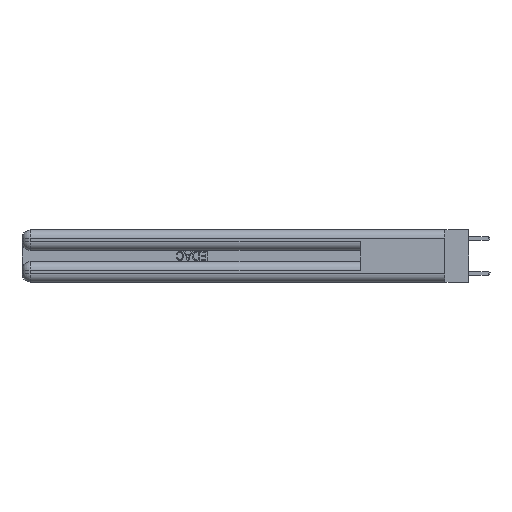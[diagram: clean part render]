
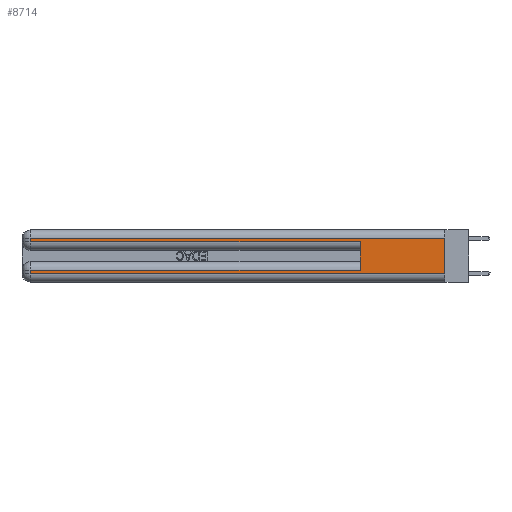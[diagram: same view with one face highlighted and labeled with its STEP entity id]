
A CAD part, left-side view. The second image highlights one B-rep face of the part: STEP entity #8714.
In plain terms, the highlighted planar face has unit normal (-1, 0, 0).
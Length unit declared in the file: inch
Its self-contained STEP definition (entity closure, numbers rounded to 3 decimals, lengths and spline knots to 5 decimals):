
#785 = CARTESIAN_POINT ( 'NONE',  ( 0., 0.6, 0.085 ) ) ;
#1132 = LINE ( 'NONE', #3684, #12643 ) ;
#1412 = CARTESIAN_POINT ( 'NONE',  ( 0., 2.94, 0.31 ) ) ;
#2000 = CARTESIAN_POINT ( 'NONE',  ( 0., 0., 0.31 ) ) ;
#2196 = DIRECTION ( 'NONE',  ( 0., -1., 0. ) ) ;
#3432 = CARTESIAN_POINT ( 'NONE',  ( 0., 0., 0.31 ) ) ;
#3684 = CARTESIAN_POINT ( 'NONE',  ( 0., 0., 0.06 ) ) ;
#5345 = EDGE_CURVE ( 'NONE', #19648, #17023, #16332, .T. ) ;
#5467 = DIRECTION ( 'NONE',  ( 1., 0., 0. ) ) ;
#5816 = DIRECTION ( 'NONE',  ( 0., 0., -1. ) ) ;
#6574 = AXIS2_PLACEMENT_3D ( 'NONE', #23707, #5467, #21513 ) ;
#6749 = CARTESIAN_POINT ( 'NONE',  ( 0., 0., 0.285 ) ) ;
#7258 = VERTEX_POINT ( 'NONE', #28825 ) ;
#8148 = VERTEX_POINT ( 'NONE', #28732 ) ;
#8714 = ADVANCED_FACE ( 'NONE', ( #24855 ), #19241, .F. ) ;
#8720 = CARTESIAN_POINT ( 'NONE',  ( 0., 2.94, 0.37 ) ) ;
#9172 = VECTOR ( 'NONE', #20385, 39.37008 ) ;
#9452 = VERTEX_POINT ( 'NONE', #3432 ) ;
#10529 = VECTOR ( 'NONE', #26042, 39.37008 ) ;
#10895 = CARTESIAN_POINT ( 'NONE',  ( 0., 0.6, 0.145 ) ) ;
#11753 = EDGE_CURVE ( 'NONE', #17023, #7258, #26459, .T. ) ;
#12235 = EDGE_CURVE ( 'NONE', #12802, #8148, #26435, .T. ) ;
#12643 = VECTOR ( 'NONE', #24319, 39.37008 ) ;
#12802 = VERTEX_POINT ( 'NONE', #21899 ) ;
#15195 = ORIENTED_EDGE ( 'NONE', *, *, #27402, .F. ) ;
#15209 = ORIENTED_EDGE ( 'NONE', *, *, #21776, .T. ) ;
#16332 = LINE ( 'NONE', #26204, #27722 ) ;
#16548 = ORIENTED_EDGE ( 'NONE', *, *, #12235, .T. ) ;
#17023 = VERTEX_POINT ( 'NONE', #24270 ) ;
#17419 = VECTOR ( 'NONE', #29164, 39.37008 ) ;
#17841 = ORIENTED_EDGE ( 'NONE', *, *, #11753, .T. ) ;
#19091 = EDGE_CURVE ( 'NONE', #25580, #7258, #24151, .T. ) ;
#19241 = PLANE ( 'NONE',  #6574 ) ;
#19560 = CARTESIAN_POINT ( 'NONE',  ( 0., 0., 0.37 ) ) ;
#19648 = VERTEX_POINT ( 'NONE', #1412 ) ;
#20385 = DIRECTION ( 'NONE',  ( 0., 1., 0. ) ) ;
#20410 = VECTOR ( 'NONE', #22418, 39.37008 ) ;
#20784 = ORIENTED_EDGE ( 'NONE', *, *, #22596, .T. ) ;
#21120 = VECTOR ( 'NONE', #2196, 39.37008 ) ;
#21513 = DIRECTION ( 'NONE',  ( 0., 0., -1. ) ) ;
#21768 = EDGE_LOOP ( 'NONE', ( #15195, #28402, #27435, #17841, #26720, #15209, #16548, #20784 ) ) ;
#21776 = EDGE_CURVE ( 'NONE', #25580, #12802, #28029, .T. ) ;
#21899 = CARTESIAN_POINT ( 'NONE',  ( 0., 2.94, 0.085 ) ) ;
#22418 = DIRECTION ( 'NONE',  ( 0., 0., -1. ) ) ;
#22596 = EDGE_CURVE ( 'NONE', #8148, #23197, #1132, .T. ) ;
#23197 = VERTEX_POINT ( 'NONE', #24958 ) ;
#23463 = VECTOR ( 'NONE', #5816, 39.37008 ) ;
#23707 = CARTESIAN_POINT ( 'NONE',  ( 0., 0., 0.37 ) ) ;
#23763 = CARTESIAN_POINT ( 'NONE',  ( 0., 0., 0.085 ) ) ;
#24151 = LINE ( 'NONE', #10895, #17419 ) ;
#24183 = LINE ( 'NONE', #19560, #23463 ) ;
#24270 = CARTESIAN_POINT ( 'NONE',  ( 0., 2.94, 0.285 ) ) ;
#24319 = DIRECTION ( 'NONE',  ( 0., -1., 0. ) ) ;
#24855 = FACE_OUTER_BOUND ( 'NONE', #21768, .T. ) ;
#24958 = CARTESIAN_POINT ( 'NONE',  ( 0., 0., 0.06 ) ) ;
#25580 = VERTEX_POINT ( 'NONE', #785 ) ;
#26042 = DIRECTION ( 'NONE',  ( 0., 1., 0. ) ) ;
#26204 = CARTESIAN_POINT ( 'NONE',  ( 0., 2.94, 0.37 ) ) ;
#26435 = LINE ( 'NONE', #8720, #20410 ) ;
#26459 = LINE ( 'NONE', #6749, #21120 ) ;
#26720 = ORIENTED_EDGE ( 'NONE', *, *, #19091, .F. ) ;
#27058 = EDGE_CURVE ( 'NONE', #9452, #19648, #27410, .T. ) ;
#27402 = EDGE_CURVE ( 'NONE', #9452, #23197, #24183, .T. ) ;
#27410 = LINE ( 'NONE', #2000, #9172 ) ;
#27435 = ORIENTED_EDGE ( 'NONE', *, *, #5345, .T. ) ;
#27722 = VECTOR ( 'NONE', #28512, 39.37008 ) ;
#28029 = LINE ( 'NONE', #23763, #10529 ) ;
#28402 = ORIENTED_EDGE ( 'NONE', *, *, #27058, .T. ) ;
#28512 = DIRECTION ( 'NONE',  ( 0., 0., -1. ) ) ;
#28732 = CARTESIAN_POINT ( 'NONE',  ( 0., 2.94, 0.06 ) ) ;
#28825 = CARTESIAN_POINT ( 'NONE',  ( 0., 0.6, 0.285 ) ) ;
#29164 = DIRECTION ( 'NONE',  ( 0., 0., 1. ) ) ;
